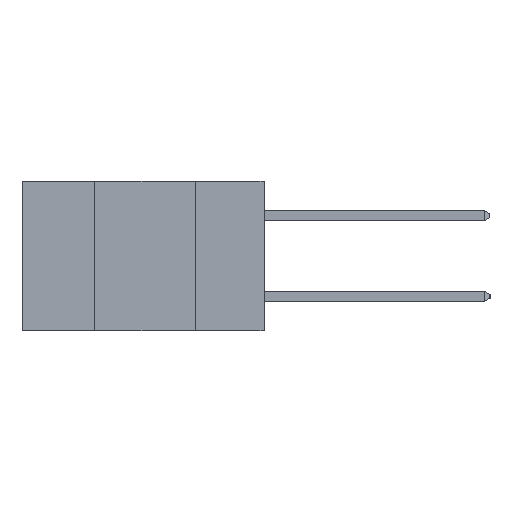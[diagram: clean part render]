
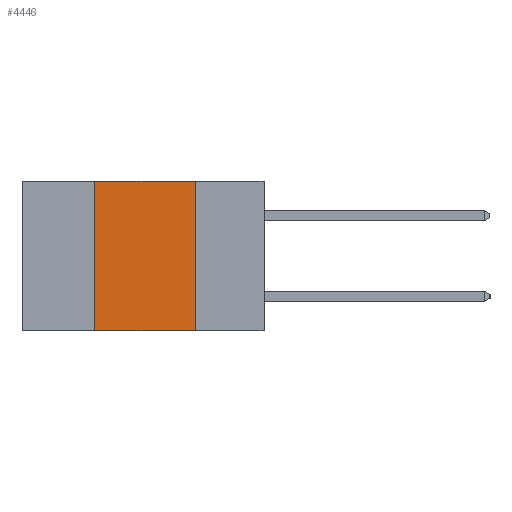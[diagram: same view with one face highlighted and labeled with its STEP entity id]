
A CAD part, left-side view. The second image highlights one B-rep face of the part: STEP entity #4446.
In plain terms, the highlighted planar face has unit normal (-1, 0, 0).
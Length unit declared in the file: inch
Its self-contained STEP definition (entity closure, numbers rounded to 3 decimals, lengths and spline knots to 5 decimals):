
#352 = DIRECTION ( 'NONE',  ( 0., 0., 1. ) ) ;
#667 = CARTESIAN_POINT ( 'NONE',  ( 0., 0.42, -0.37 ) ) ;
#751 = VECTOR ( 'NONE', #352, 39.37008 ) ;
#1566 = VERTEX_POINT ( 'NONE', #14700 ) ;
#1722 = VECTOR ( 'NONE', #4655, 39.37008 ) ;
#2181 = CARTESIAN_POINT ( 'NONE',  ( 0., 0.17, -0.37 ) ) ;
#2512 = ORIENTED_EDGE ( 'NONE', *, *, #6453, .F. ) ;
#2895 = AXIS2_PLACEMENT_3D ( 'NONE', #11716, #11666, #11590 ) ;
#3210 = FACE_OUTER_BOUND ( 'NONE', #14938, .T. ) ;
#3299 = ORIENTED_EDGE ( 'NONE', *, *, #3979, .T. ) ;
#3626 = LINE ( 'NONE', #16049, #13666 ) ;
#3979 = EDGE_CURVE ( 'NONE', #13955, #11657, #3626, .T. ) ;
#4050 = DIRECTION ( 'NONE',  ( 0., 0., -1. ) ) ;
#4446 = ADVANCED_FACE ( 'NONE', ( #3210 ), #11720, .F. ) ;
#4655 = DIRECTION ( 'NONE',  ( 0., -1., 0. ) ) ;
#5686 = VECTOR ( 'NONE', #4050, 39.37008 ) ;
#5796 = EDGE_CURVE ( 'NONE', #8804, #11657, #9840, .T. ) ;
#6453 = EDGE_CURVE ( 'NONE', #13955, #1566, #9623, .T. ) ;
#7756 = CARTESIAN_POINT ( 'NONE',  ( 0., 0.17, -0.37 ) ) ;
#8804 = VERTEX_POINT ( 'NONE', #11670 ) ;
#9623 = LINE ( 'NONE', #11734, #751 ) ;
#9840 = LINE ( 'NONE', #7756, #5686 ) ;
#10577 = ORIENTED_EDGE ( 'NONE', *, *, #5796, .F. ) ;
#10926 = CARTESIAN_POINT ( 'NONE',  ( 0., 0.6, 0. ) ) ;
#11354 = ORIENTED_EDGE ( 'NONE', *, *, #11632, .F. ) ;
#11590 = DIRECTION ( 'NONE',  ( 0., 0., -1. ) ) ;
#11632 = EDGE_CURVE ( 'NONE', #1566, #8804, #15151, .T. ) ;
#11657 = VERTEX_POINT ( 'NONE', #2181 ) ;
#11666 = DIRECTION ( 'NONE',  ( 1., 0., 0. ) ) ;
#11670 = CARTESIAN_POINT ( 'NONE',  ( 0., 0.17, 0. ) ) ;
#11716 = CARTESIAN_POINT ( 'NONE',  ( 0., 0.6, 0. ) ) ;
#11720 = PLANE ( 'NONE',  #2895 ) ;
#11734 = CARTESIAN_POINT ( 'NONE',  ( 0., 0.42, -0.37 ) ) ;
#13666 = VECTOR ( 'NONE', #16213, 39.37008 ) ;
#13955 = VERTEX_POINT ( 'NONE', #667 ) ;
#14700 = CARTESIAN_POINT ( 'NONE',  ( 0., 0.42, 0. ) ) ;
#14938 = EDGE_LOOP ( 'NONE', ( #10577, #11354, #2512, #3299 ) ) ;
#15151 = LINE ( 'NONE', #10926, #1722 ) ;
#16049 = CARTESIAN_POINT ( 'NONE',  ( 0., 0.6, -0.37 ) ) ;
#16213 = DIRECTION ( 'NONE',  ( 0., -1., 0. ) ) ;
